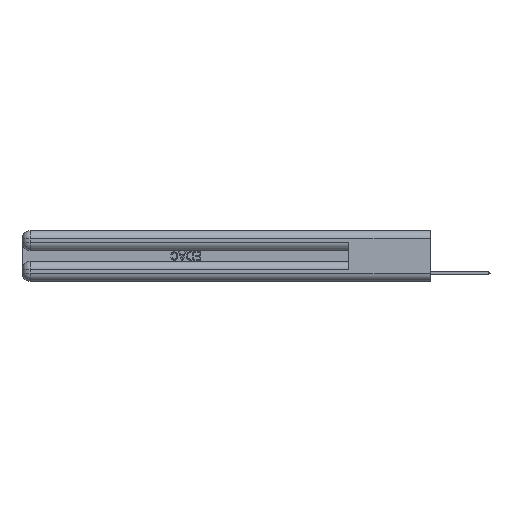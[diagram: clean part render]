
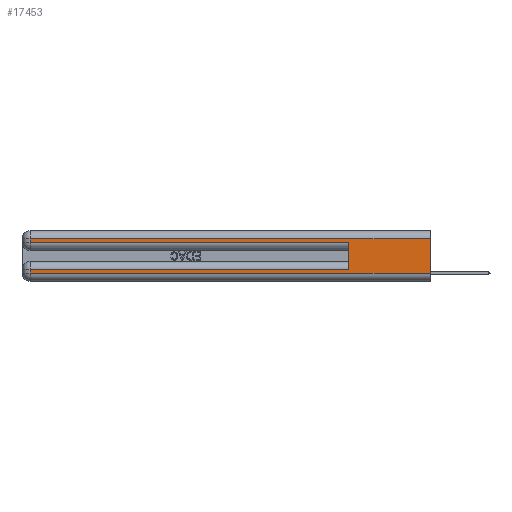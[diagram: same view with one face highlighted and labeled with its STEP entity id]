
A CAD part, left-side view. The second image highlights one B-rep face of the part: STEP entity #17453.
In plain terms, the highlighted planar face has unit normal (-1, 0, 0).
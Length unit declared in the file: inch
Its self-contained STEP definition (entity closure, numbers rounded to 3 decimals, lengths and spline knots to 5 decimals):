
#156 = LINE ( 'NONE', #12289, #24336 ) ;
#470 = EDGE_CURVE ( 'NONE', #1210, #9043, #17519, .T. ) ;
#717 = VECTOR ( 'NONE', #5161, 39.37008 ) ;
#1210 = VERTEX_POINT ( 'NONE', #25873 ) ;
#1793 = VECTOR ( 'NONE', #4261, 39.37008 ) ;
#2332 = EDGE_CURVE ( 'NONE', #7959, #27528, #8818, .T. ) ;
#2507 = CARTESIAN_POINT ( 'NONE',  ( 0., 0., 0.085 ) ) ;
#3927 = CARTESIAN_POINT ( 'NONE',  ( 0., 0., 0.06 ) ) ;
#4261 = DIRECTION ( 'NONE',  ( 0., 1., 0. ) ) ;
#4328 = VECTOR ( 'NONE', #24668, 39.37008 ) ;
#4578 = LINE ( 'NONE', #2507, #1793 ) ;
#4926 = ORIENTED_EDGE ( 'NONE', *, *, #30308, .T. ) ;
#5161 = DIRECTION ( 'NONE',  ( 0., 0., -1. ) ) ;
#5830 = ORIENTED_EDGE ( 'NONE', *, *, #29044, .T. ) ;
#5924 = VERTEX_POINT ( 'NONE', #24858 ) ;
#6085 = VERTEX_POINT ( 'NONE', #9051 ) ;
#6176 = VECTOR ( 'NONE', #30559, 39.37008 ) ;
#6416 = CARTESIAN_POINT ( 'NONE',  ( 0., 0., 0.285 ) ) ;
#7667 = EDGE_CURVE ( 'NONE', #6085, #27528, #15298, .T. ) ;
#7701 = DIRECTION ( 'NONE',  ( 1., 0., 0. ) ) ;
#7959 = VERTEX_POINT ( 'NONE', #27177 ) ;
#8818 = LINE ( 'NONE', #3927, #23167 ) ;
#9009 = ORIENTED_EDGE ( 'NONE', *, *, #470, .T. ) ;
#9018 = DIRECTION ( 'NONE',  ( 0., 0., 1. ) ) ;
#9043 = VERTEX_POINT ( 'NONE', #27603 ) ;
#9051 = CARTESIAN_POINT ( 'NONE',  ( 0., 0., 0.31 ) ) ;
#9088 = LINE ( 'NONE', #6416, #6176 ) ;
#10294 = VERTEX_POINT ( 'NONE', #26393 ) ;
#10534 = FACE_OUTER_BOUND ( 'NONE', #14040, .T. ) ;
#10639 = VECTOR ( 'NONE', #27055, 39.37008 ) ;
#11168 = DIRECTION ( 'NONE',  ( 0., -1., 0. ) ) ;
#11851 = ORIENTED_EDGE ( 'NONE', *, *, #26683, .T. ) ;
#12289 = CARTESIAN_POINT ( 'NONE',  ( 0., 0., 0.31 ) ) ;
#14040 = EDGE_LOOP ( 'NONE', ( #24148, #24147, #9009, #11851, #29292, #4926, #5830, #27547 ) ) ;
#14647 = DIRECTION ( 'NONE',  ( 0., 1., 0. ) ) ;
#14980 = CARTESIAN_POINT ( 'NONE',  ( 0., 2.94, 0.37 ) ) ;
#14983 = CARTESIAN_POINT ( 'NONE',  ( 0., 0., 0.06 ) ) ;
#15298 = LINE ( 'NONE', #24982, #10639 ) ;
#16232 = LINE ( 'NONE', #18286, #23359 ) ;
#17453 = ADVANCED_FACE ( 'NONE', ( #10534 ), #24297, .F. ) ;
#17519 = LINE ( 'NONE', #14980, #4328 ) ;
#18216 = EDGE_CURVE ( 'NONE', #6085, #1210, #156, .T. ) ;
#18286 = CARTESIAN_POINT ( 'NONE',  ( 0., 0.6, 0.145 ) ) ;
#21216 = CARTESIAN_POINT ( 'NONE',  ( 0., 0.6, 0.285 ) ) ;
#23167 = VECTOR ( 'NONE', #11168, 39.37008 ) ;
#23359 = VECTOR ( 'NONE', #9018, 39.37008 ) ;
#24147 = ORIENTED_EDGE ( 'NONE', *, *, #18216, .T. ) ;
#24148 = ORIENTED_EDGE ( 'NONE', *, *, #7667, .F. ) ;
#24263 = LINE ( 'NONE', #26786, #717 ) ;
#24297 = PLANE ( 'NONE',  #29838 ) ;
#24336 = VECTOR ( 'NONE', #14647, 39.37008 ) ;
#24668 = DIRECTION ( 'NONE',  ( 0., 0., -1. ) ) ;
#24858 = CARTESIAN_POINT ( 'NONE',  ( 0., 0.6, 0.085 ) ) ;
#24982 = CARTESIAN_POINT ( 'NONE',  ( 0., 0., 0.37 ) ) ;
#25873 = CARTESIAN_POINT ( 'NONE',  ( 0., 2.94, 0.31 ) ) ;
#26393 = CARTESIAN_POINT ( 'NONE',  ( 0., 2.94, 0.085 ) ) ;
#26668 = VERTEX_POINT ( 'NONE', #21216 ) ;
#26683 = EDGE_CURVE ( 'NONE', #9043, #26668, #9088, .T. ) ;
#26786 = CARTESIAN_POINT ( 'NONE',  ( 0., 2.94, 0.37 ) ) ;
#26985 = CARTESIAN_POINT ( 'NONE',  ( 0., 0., 0.37 ) ) ;
#27055 = DIRECTION ( 'NONE',  ( 0., 0., -1. ) ) ;
#27148 = DIRECTION ( 'NONE',  ( 0., 0., -1. ) ) ;
#27177 = CARTESIAN_POINT ( 'NONE',  ( 0., 2.94, 0.06 ) ) ;
#27528 = VERTEX_POINT ( 'NONE', #14983 ) ;
#27547 = ORIENTED_EDGE ( 'NONE', *, *, #2332, .T. ) ;
#27603 = CARTESIAN_POINT ( 'NONE',  ( 0., 2.94, 0.285 ) ) ;
#27628 = EDGE_CURVE ( 'NONE', #5924, #26668, #16232, .T. ) ;
#29044 = EDGE_CURVE ( 'NONE', #10294, #7959, #24263, .T. ) ;
#29292 = ORIENTED_EDGE ( 'NONE', *, *, #27628, .F. ) ;
#29838 = AXIS2_PLACEMENT_3D ( 'NONE', #26985, #7701, #27148 ) ;
#30308 = EDGE_CURVE ( 'NONE', #5924, #10294, #4578, .T. ) ;
#30559 = DIRECTION ( 'NONE',  ( 0., -1., 0. ) ) ;
